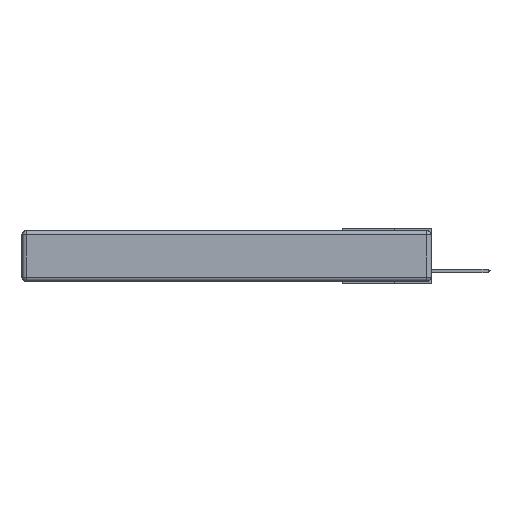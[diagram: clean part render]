
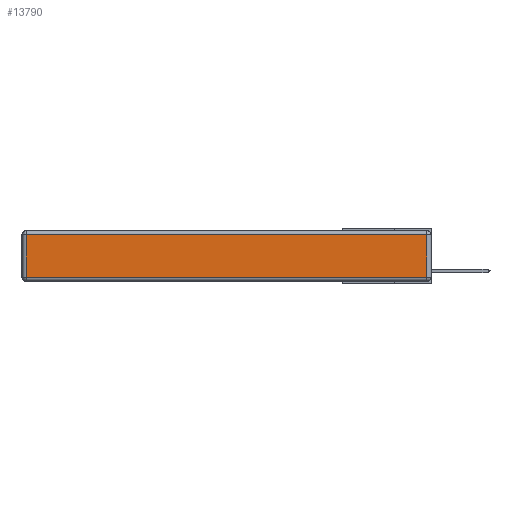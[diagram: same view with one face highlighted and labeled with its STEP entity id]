
A CAD part, left-side view. The second image highlights one B-rep face of the part: STEP entity #13790.
In plain terms, the highlighted planar face has unit normal (-1, 0, 0).
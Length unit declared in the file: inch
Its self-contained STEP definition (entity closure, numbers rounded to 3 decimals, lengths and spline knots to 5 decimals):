
#256 = ORIENTED_EDGE ( 'NONE', *, *, #17288, .T. ) ;
#763 = CARTESIAN_POINT ( 'NONE',  ( 0., 0.03, -0.03 ) ) ;
#903 = DIRECTION ( 'NONE',  ( -1., 0., 0. ) ) ;
#1168 = EDGE_CURVE ( 'NONE', #12792, #13779, #2724, .T. ) ;
#2724 = LINE ( 'NONE', #16051, #19065 ) ;
#2846 = EDGE_LOOP ( 'NONE', ( #7533, #7726, #256, #19839 ) ) ;
#3217 = AXIS2_PLACEMENT_3D ( 'NONE', #16175, #903, #16305 ) ;
#3610 = VERTEX_POINT ( 'NONE', #6504 ) ;
#3958 = LINE ( 'NONE', #17566, #11869 ) ;
#5251 = FACE_OUTER_BOUND ( 'NONE', #2846, .T. ) ;
#5283 = DIRECTION ( 'NONE',  ( 0., 0., 1. ) ) ;
#6504 = CARTESIAN_POINT ( 'NONE',  ( 0., 2.72, -0.313 ) ) ;
#7533 = ORIENTED_EDGE ( 'NONE', *, *, #12399, .T. ) ;
#7726 = ORIENTED_EDGE ( 'NONE', *, *, #1168, .T. ) ;
#9032 = VECTOR ( 'NONE', #10954, 39.37008 ) ;
#9237 = CARTESIAN_POINT ( 'NONE',  ( 0., 2.72, -0.03 ) ) ;
#10954 = DIRECTION ( 'NONE',  ( 0., 0., -1. ) ) ;
#11011 = VECTOR ( 'NONE', #14473, 39.37008 ) ;
#11086 = CARTESIAN_POINT ( 'NONE',  ( 0., 2.72, -0.343 ) ) ;
#11713 = LINE ( 'NONE', #12486, #11011 ) ;
#11869 = VECTOR ( 'NONE', #14376, 39.37008 ) ;
#12186 = CARTESIAN_POINT ( 'NONE',  ( 0., 0.03, -0.313 ) ) ;
#12399 = EDGE_CURVE ( 'NONE', #3610, #12792, #11713, .T. ) ;
#12486 = CARTESIAN_POINT ( 'NONE',  ( 0., 0., -0.313 ) ) ;
#12792 = VERTEX_POINT ( 'NONE', #12186 ) ;
#13361 = LINE ( 'NONE', #11086, #9032 ) ;
#13419 = EDGE_CURVE ( 'NONE', #16281, #3610, #13361, .T. ) ;
#13779 = VERTEX_POINT ( 'NONE', #763 ) ;
#13790 = ADVANCED_FACE ( 'NONE', ( #5251 ), #14624, .T. ) ;
#14376 = DIRECTION ( 'NONE',  ( 0., 1., 0. ) ) ;
#14473 = DIRECTION ( 'NONE',  ( 0., -1., 0. ) ) ;
#14624 = PLANE ( 'NONE',  #3217 ) ;
#16051 = CARTESIAN_POINT ( 'NONE',  ( 0., 0.03, -0.343 ) ) ;
#16175 = CARTESIAN_POINT ( 'NONE',  ( 0., 0., -0.343 ) ) ;
#16281 = VERTEX_POINT ( 'NONE', #9237 ) ;
#16305 = DIRECTION ( 'NONE',  ( 0., 0., 1. ) ) ;
#17288 = EDGE_CURVE ( 'NONE', #13779, #16281, #3958, .T. ) ;
#17566 = CARTESIAN_POINT ( 'NONE',  ( 0., 2.75, -0.03 ) ) ;
#19065 = VECTOR ( 'NONE', #5283, 39.37008 ) ;
#19839 = ORIENTED_EDGE ( 'NONE', *, *, #13419, .T. ) ;
